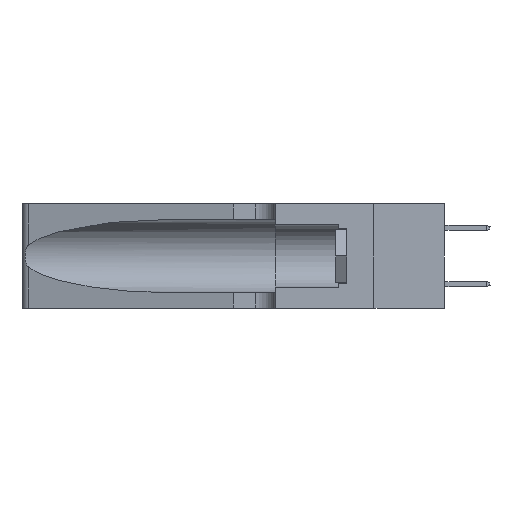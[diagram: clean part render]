
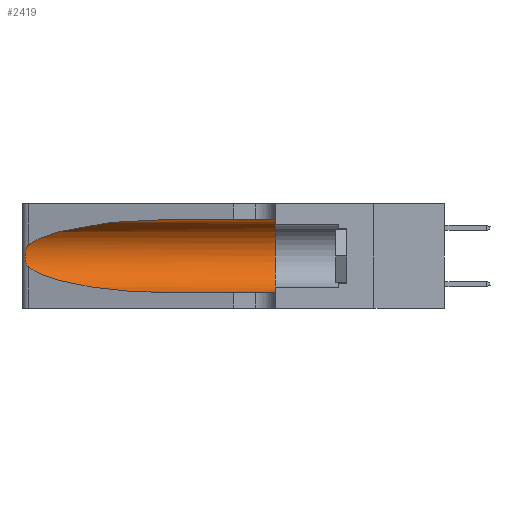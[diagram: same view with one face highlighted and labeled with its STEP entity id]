
A CAD part, left-side view. The second image highlights one B-rep face of the part: STEP entity #2419.
In plain terms, the highlighted cylindrical face has radius 3.308 mm (diameter 6.617 mm), a partial arc.
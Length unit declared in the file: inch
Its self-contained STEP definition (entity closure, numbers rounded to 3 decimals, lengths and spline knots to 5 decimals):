
#565 = CARTESIAN_POINT ( 'NONE',  ( 0.26075, 1.23896, 0.178 ) ) ;
#1279 = CARTESIAN_POINT ( 'NONE',  ( 0.1305, 1.61858, 0.185 ) ) ;
#1511 = VERTEX_POINT ( 'NONE', #18599 ) ;
#1529 = VECTOR ( 'NONE', #13262, 39.37008 ) ;
#1680 = CARTESIAN_POINT ( 'NONE',  ( 0.1305, 1.61858, 0.05475 ) ) ;
#2117 = CARTESIAN_POINT ( 'NONE',  ( 0.25856, 1.23593, 0.16098 ) ) ;
#2419 = ADVANCED_FACE ( 'NONE', ( #11286 ), #18817, .F. ) ;
#2750 = EDGE_CURVE ( 'NONE', #5478, #15810, #13615, .T. ) ;
#3643 = CARTESIAN_POINT ( 'NONE',  ( 0.25639, 1.23186, 0.15144 ) ) ;
#4439 = CARTESIAN_POINT ( 'NONE',  ( 0.18966, 0.96281, 0.05475 ) ) ;
#5157 = CARTESIAN_POINT ( 'NONE',  ( 0.25487, 1.22718, 0.14631 ) ) ;
#5189 = DIRECTION ( 'NONE',  ( 0., -1., 0. ) ) ;
#5478 = VERTEX_POINT ( 'NONE', #10628 ) ;
#6088 = DIRECTION ( 'NONE',  ( 0., 1., 0. ) ) ;
#6324 = DIRECTION ( 'NONE',  ( 0., 0., -1. ) ) ;
#6500 = CARTESIAN_POINT ( 'NONE',  ( 0.25487, 1.22718, 0.22369 ) ) ;
#6627 = CARTESIAN_POINT ( 'NONE',  ( 0.25639, 1.23184, 0.21858 ) ) ;
#6824 = EDGE_CURVE ( 'NONE', #1511, #16547, #10815, .T. ) ;
#6989 = CARTESIAN_POINT ( 'NONE',  ( 0.1305, 0.72297, 0.31525 ) ) ;
#7221 = CARTESIAN_POINT ( 'NONE',  ( 0.1305, 0.35, 0.05475 ) ) ;
#7546 = EDGE_CURVE ( 'NONE', #16547, #14954, #8027, .T. ) ;
#7888 = EDGE_CURVE ( 'NONE', #5478, #14618, #11827, .T. ) ;
#8027 = LINE ( 'NONE', #1680, #15551 ) ;
#8057 = ORIENTED_EDGE ( 'NONE', *, *, #7546, .T. ) ;
#8146 = CARTESIAN_POINT ( 'NONE',  ( 0.25854, 1.2359, 0.20912 ) ) ;
#8513 = CARTESIAN_POINT ( 'NONE',  ( 0.2373, 1.15595, 0.28018 ) ) ;
#9685 = CARTESIAN_POINT ( 'NONE',  ( 0.26075, 1.23896, 0.19203 ) ) ;
#10481 = CARTESIAN_POINT ( 'NONE',  ( 0.25487, 1.22718, 0.14631 ) ) ;
#10628 = CARTESIAN_POINT ( 'NONE',  ( 0.1305, 0.72297, 0.31525 ) ) ;
#10815 =( BOUNDED_CURVE ( )  B_SPLINE_CURVE ( 3, ( #10481, #19493, #4439, #14973 ),
 .UNSPECIFIED., .F., .F. ) 
 B_SPLINE_CURVE_WITH_KNOTS ( ( 4, 4 ),
 ( 3.44316, 4.71239 ),
 .UNSPECIFIED. ) 
 CURVE ( )  GEOMETRIC_REPRESENTATION_ITEM ( )  RATIONAL_B_SPLINE_CURVE ( ( 1., 0.87, 0.87, 1. ) ) 
 REPRESENTATION_ITEM ( '' )  );
#11139 = CARTESIAN_POINT ( 'NONE',  ( 0.25487, 1.22718, 0.22369 ) ) ;
#11200 = CARTESIAN_POINT ( 'NONE',  ( 0.26017, 1.23833, 0.17102 ) ) ;
#11205 = AXIS2_PLACEMENT_3D ( 'NONE', #15100, #6088, #16624 ) ;
#11286 = FACE_OUTER_BOUND ( 'NONE', #16210, .T. ) ;
#11827 =( BOUNDED_CURVE ( )  B_SPLINE_CURVE ( 3, ( #6989, #13001, #8513, #19052 ),
 .UNSPECIFIED., .F., .T. ) 
 B_SPLINE_CURVE_WITH_KNOTS ( ( 4, 4 ),
 ( 1.5708, 2.84003 ),
 .UNSPECIFIED. ) 
 CURVE ( )  GEOMETRIC_REPRESENTATION_ITEM ( )  RATIONAL_B_SPLINE_CURVE ( ( 1., 0.87, 0.87, 1. ) ) 
 REPRESENTATION_ITEM ( '' )  );
#12593 = CIRCLE ( 'NONE', #11205, 0.13025 ) ;
#12711 = CARTESIAN_POINT ( 'NONE',  ( 0.25789, 1.23486, 0.15765 ) ) ;
#12865 = B_SPLINE_CURVE_WITH_KNOTS ( 'NONE', 3,
 ( #11139, #18632, #6627, #17178, #8146, #18703, #9685, #565, #11200, #2117, #12711, #3643, #14213, #5157 ),
 .UNSPECIFIED., .F., .F.,
 ( 4, 2, 2, 2, 2, 2, 4 ),
 ( 0., 0.00027, 0.00053, 0.00107, 0.0016, 0.00187, 0.00214 ),
 .UNSPECIFIED. ) ;
#12900 = EDGE_CURVE ( 'NONE', #14618, #1511, #12865, .T. ) ;
#13001 = CARTESIAN_POINT ( 'NONE',  ( 0.18966, 0.96281, 0.31525 ) ) ;
#13077 = ORIENTED_EDGE ( 'NONE', *, *, #7888, .T. ) ;
#13262 = DIRECTION ( 'NONE',  ( 0., -1., 0. ) ) ;
#13615 = LINE ( 'NONE', #18238, #1529 ) ;
#14213 = CARTESIAN_POINT ( 'NONE',  ( 0.25555, 1.22993, 0.14849 ) ) ;
#14316 = CARTESIAN_POINT ( 'NONE',  ( 0.1305, 0.72297, 0.05475 ) ) ;
#14566 = AXIS2_PLACEMENT_3D ( 'NONE', #1279, #5189, #6324 ) ;
#14618 = VERTEX_POINT ( 'NONE', #6500 ) ;
#14954 = VERTEX_POINT ( 'NONE', #7221 ) ;
#14973 = CARTESIAN_POINT ( 'NONE',  ( 0.1305, 0.72297, 0.05475 ) ) ;
#15100 = CARTESIAN_POINT ( 'NONE',  ( 0.1305, 0.35, 0.185 ) ) ;
#15551 = VECTOR ( 'NONE', #16739, 39.37008 ) ;
#15810 = VERTEX_POINT ( 'NONE', #17183 ) ;
#16210 = EDGE_LOOP ( 'NONE', ( #13077, #17709, #18604, #8057, #19596, #19509 ) ) ;
#16547 = VERTEX_POINT ( 'NONE', #14316 ) ;
#16624 = DIRECTION ( 'NONE',  ( 0., 0., 1. ) ) ;
#16739 = DIRECTION ( 'NONE',  ( 0., -1., 0. ) ) ;
#17178 = CARTESIAN_POINT ( 'NONE',  ( 0.25787, 1.23484, 0.2124 ) ) ;
#17183 = CARTESIAN_POINT ( 'NONE',  ( 0.1305, 0.35, 0.31525 ) ) ;
#17709 = ORIENTED_EDGE ( 'NONE', *, *, #12900, .T. ) ;
#18238 = CARTESIAN_POINT ( 'NONE',  ( 0.1305, 1.61858, 0.31525 ) ) ;
#18599 = CARTESIAN_POINT ( 'NONE',  ( 0.25487, 1.22718, 0.14631 ) ) ;
#18604 = ORIENTED_EDGE ( 'NONE', *, *, #6824, .T. ) ;
#18632 = CARTESIAN_POINT ( 'NONE',  ( 0.25555, 1.22994, 0.2215 ) ) ;
#18703 = CARTESIAN_POINT ( 'NONE',  ( 0.26018, 1.23835, 0.19895 ) ) ;
#18817 = CYLINDRICAL_SURFACE ( 'NONE', #14566, 0.13025 ) ;
#19052 = CARTESIAN_POINT ( 'NONE',  ( 0.25487, 1.22718, 0.22369 ) ) ;
#19477 = EDGE_CURVE ( 'NONE', #15810, #14954, #12593, .T. ) ;
#19493 = CARTESIAN_POINT ( 'NONE',  ( 0.2373, 1.15595, 0.08982 ) ) ;
#19509 = ORIENTED_EDGE ( 'NONE', *, *, #2750, .F. ) ;
#19596 = ORIENTED_EDGE ( 'NONE', *, *, #19477, .F. ) ;
